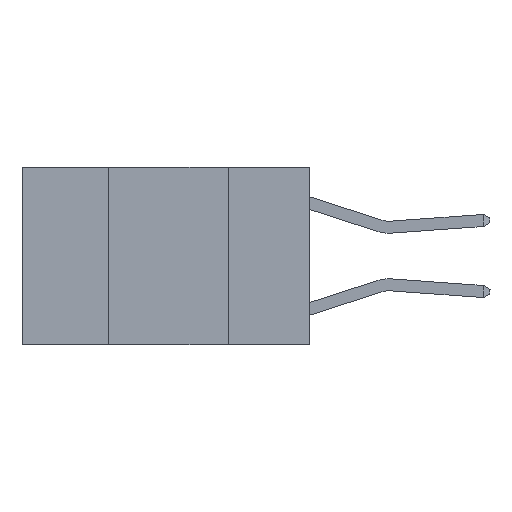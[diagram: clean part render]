
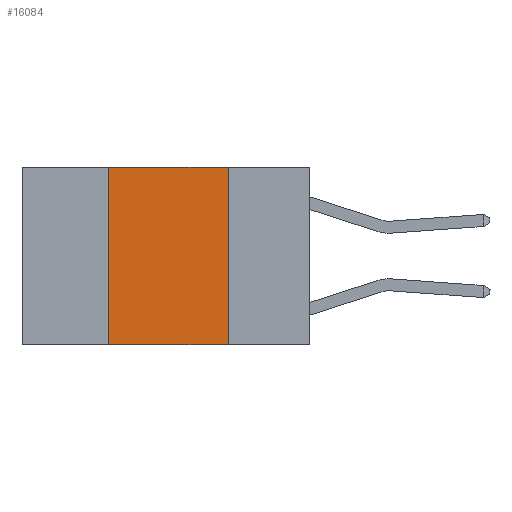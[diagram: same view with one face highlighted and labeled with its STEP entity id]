
A CAD part, left-side view. The second image highlights one B-rep face of the part: STEP entity #16084.
In plain terms, the highlighted planar face has unit normal (-1, 0, 0).
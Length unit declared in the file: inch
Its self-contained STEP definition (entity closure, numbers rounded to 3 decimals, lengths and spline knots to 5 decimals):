
#633 = CARTESIAN_POINT ( 'NONE',  ( 0., 0.6, -0.37 ) ) ;
#1813 = EDGE_CURVE ( 'NONE', #5357, #18060, #15093, .T. ) ;
#1858 = CARTESIAN_POINT ( 'NONE',  ( 0., 0.17, 0. ) ) ;
#2096 = VERTEX_POINT ( 'NONE', #1858 ) ;
#2243 = DIRECTION ( 'NONE',  ( 0., -1., 0. ) ) ;
#3214 = EDGE_CURVE ( 'NONE', #18060, #2096, #27216, .T. ) ;
#3481 = VECTOR ( 'NONE', #7675, 39.37008 ) ;
#4088 = EDGE_CURVE ( 'NONE', #5357, #26430, #23327, .T. ) ;
#5095 = CARTESIAN_POINT ( 'NONE',  ( 0., 0.17, 0. ) ) ;
#5357 = VERTEX_POINT ( 'NONE', #12948 ) ;
#6159 = CARTESIAN_POINT ( 'NONE',  ( 0., 0.42, 0. ) ) ;
#6961 = CARTESIAN_POINT ( 'NONE',  ( 0., 0.6, 0. ) ) ;
#7675 = DIRECTION ( 'NONE',  ( 0., 0., -1. ) ) ;
#8537 = EDGE_LOOP ( 'NONE', ( #12033, #21692, #9497, #28023 ) ) ;
#8704 = VECTOR ( 'NONE', #28544, 39.37008 ) ;
#9497 = ORIENTED_EDGE ( 'NONE', *, *, #1813, .F. ) ;
#12033 = ORIENTED_EDGE ( 'NONE', *, *, #25136, .F. ) ;
#12053 = AXIS2_PLACEMENT_3D ( 'NONE', #28801, #14087, #26205 ) ;
#12948 = CARTESIAN_POINT ( 'NONE',  ( 0., 0.42, -0.37 ) ) ;
#13930 = PLANE ( 'NONE',  #12053 ) ;
#14087 = DIRECTION ( 'NONE',  ( 1., 0., 0. ) ) ;
#14564 = VECTOR ( 'NONE', #25063, 39.37008 ) ;
#14937 = CARTESIAN_POINT ( 'NONE',  ( 0., 0.42, 0. ) ) ;
#15093 = LINE ( 'NONE', #14937, #14564 ) ;
#16084 = ADVANCED_FACE ( 'NONE', ( #16407 ), #13930, .F. ) ;
#16407 = FACE_OUTER_BOUND ( 'NONE', #8537, .T. ) ;
#18060 = VERTEX_POINT ( 'NONE', #6159 ) ;
#21692 = ORIENTED_EDGE ( 'NONE', *, *, #3214, .F. ) ;
#22440 = LINE ( 'NONE', #5095, #3481 ) ;
#22881 = CARTESIAN_POINT ( 'NONE',  ( 0., 0.17, -0.37 ) ) ;
#23200 = VECTOR ( 'NONE', #2243, 39.37008 ) ;
#23327 = LINE ( 'NONE', #633, #8704 ) ;
#25063 = DIRECTION ( 'NONE',  ( 0., 0., 1. ) ) ;
#25136 = EDGE_CURVE ( 'NONE', #2096, #26430, #22440, .T. ) ;
#26205 = DIRECTION ( 'NONE',  ( 0., 0., -1. ) ) ;
#26430 = VERTEX_POINT ( 'NONE', #22881 ) ;
#27216 = LINE ( 'NONE', #6961, #23200 ) ;
#28023 = ORIENTED_EDGE ( 'NONE', *, *, #4088, .T. ) ;
#28544 = DIRECTION ( 'NONE',  ( 0., -1., 0. ) ) ;
#28801 = CARTESIAN_POINT ( 'NONE',  ( 0., 0.6, 0. ) ) ;
